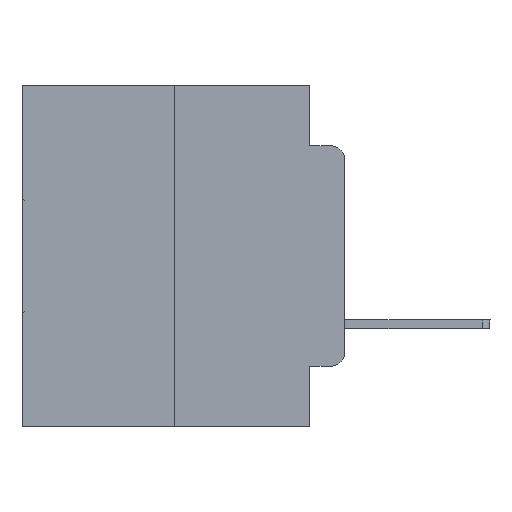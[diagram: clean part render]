
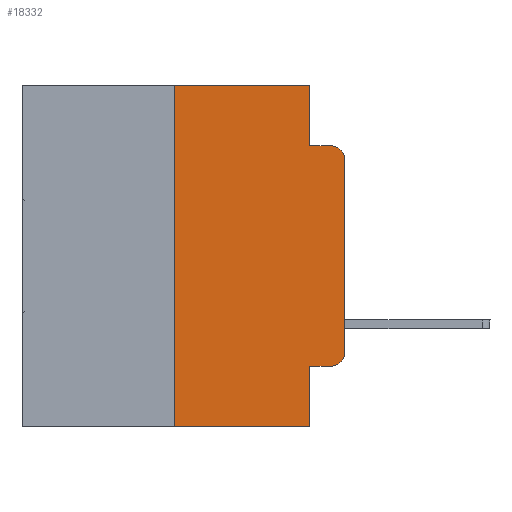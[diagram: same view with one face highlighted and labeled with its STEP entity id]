
A CAD part, left-side view. The second image highlights one B-rep face of the part: STEP entity #18332.
In plain terms, the highlighted planar face has unit normal (-1, 0, 0).
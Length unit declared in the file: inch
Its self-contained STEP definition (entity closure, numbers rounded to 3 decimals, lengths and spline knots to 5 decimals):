
#1055 = ORIENTED_EDGE ( 'NONE', *, *, #14355, .T. ) ;
#1370 = ORIENTED_EDGE ( 'NONE', *, *, #20390, .F. ) ;
#1489 = LINE ( 'NONE', #26837, #17489 ) ;
#1559 = VERTEX_POINT ( 'NONE', #23065 ) ;
#1887 = CARTESIAN_POINT ( 'NONE',  ( 0., 0.051, -0.4115 ) ) ;
#1911 = EDGE_CURVE ( 'NONE', #10479, #4880, #21654, .T. ) ;
#2182 = DIRECTION ( 'NONE',  ( 0., 0., -1. ) ) ;
#3008 = FACE_OUTER_BOUND ( 'NONE', #17630, .T. ) ;
#3124 = DIRECTION ( 'NONE',  ( 0., 0., -1. ) ) ;
#3293 = DIRECTION ( 'NONE',  ( 0., -1., 0. ) ) ;
#3843 = ORIENTED_EDGE ( 'NONE', *, *, #15880, .T. ) ;
#4880 = VERTEX_POINT ( 'NONE', #10643 ) ;
#5521 = CARTESIAN_POINT ( 'NONE',  ( 0., 0.051, -0.5 ) ) ;
#5794 = DIRECTION ( 'NONE',  ( 0., 0., 1. ) ) ;
#5913 = CARTESIAN_POINT ( 'NONE',  ( 0., 0., -0.1085 ) ) ;
#6404 = CARTESIAN_POINT ( 'NONE',  ( 0., 0.02, -0.1085 ) ) ;
#6795 = LINE ( 'NONE', #13493, #24211 ) ;
#7030 = DIRECTION ( 'NONE',  ( 1., 0., 0. ) ) ;
#7141 = DIRECTION ( 'NONE',  ( 0., -1., 0. ) ) ;
#7859 = ORIENTED_EDGE ( 'NONE', *, *, #23474, .F. ) ;
#8102 = AXIS2_PLACEMENT_3D ( 'NONE', #24826, #7030, #2182 ) ;
#8196 = ORIENTED_EDGE ( 'NONE', *, *, #9827, .F. ) ;
#8483 = EDGE_CURVE ( 'NONE', #16882, #14150, #1489, .T. ) ;
#8711 = DIRECTION ( 'NONE',  ( -1., 0., 0. ) ) ;
#9406 = VERTEX_POINT ( 'NONE', #26937 ) ;
#9827 = EDGE_CURVE ( 'NONE', #4880, #22432, #14469, .T. ) ;
#10022 = VECTOR ( 'NONE', #5794, 39.37008 ) ;
#10479 = VERTEX_POINT ( 'NONE', #19181 ) ;
#10643 = CARTESIAN_POINT ( 'NONE',  ( 0., 0.051, -0.0885 ) ) ;
#11920 = VERTEX_POINT ( 'NONE', #29093 ) ;
#12376 = CARTESIAN_POINT ( 'NONE',  ( 0., 0., 0. ) ) ;
#12474 = DIRECTION ( 'NONE',  ( 0., -1., 0. ) ) ;
#12722 = VECTOR ( 'NONE', #7141, 39.37008 ) ;
#12760 = ORIENTED_EDGE ( 'NONE', *, *, #19668, .T. ) ;
#12940 = DIRECTION ( 'NONE',  ( 0., 0., -1. ) ) ;
#13493 = CARTESIAN_POINT ( 'NONE',  ( 0., 0.051, 0. ) ) ;
#14150 = VERTEX_POINT ( 'NONE', #21867 ) ;
#14355 = EDGE_CURVE ( 'NONE', #11920, #16668, #24159, .T. ) ;
#14469 = LINE ( 'NONE', #20763, #12722 ) ;
#14696 = ORIENTED_EDGE ( 'NONE', *, *, #1911, .F. ) ;
#15263 = DIRECTION ( 'NONE',  ( 0., -1., 0. ) ) ;
#15433 = VERTEX_POINT ( 'NONE', #5521 ) ;
#15880 = EDGE_CURVE ( 'NONE', #16668, #22432, #24783, .T. ) ;
#16668 = VERTEX_POINT ( 'NONE', #5913 ) ;
#16882 = VERTEX_POINT ( 'NONE', #1887 ) ;
#17130 = CARTESIAN_POINT ( 'NONE',  ( 0., 0.25, 0. ) ) ;
#17324 = ORIENTED_EDGE ( 'NONE', *, *, #8483, .T. ) ;
#17489 = VECTOR ( 'NONE', #15263, 39.37008 ) ;
#17528 = ORIENTED_EDGE ( 'NONE', *, *, #24005, .F. ) ;
#17630 = EDGE_LOOP ( 'NONE', ( #1055, #3843, #8196, #14696, #17528, #7859, #12760, #1370, #17324, #22551 ) ) ;
#18091 = PLANE ( 'NONE',  #8102 ) ;
#18212 = AXIS2_PLACEMENT_3D ( 'NONE', #25520, #18786, #21042 ) ;
#18332 = ADVANCED_FACE ( 'NONE', ( #3008 ), #18091, .F. ) ;
#18786 = DIRECTION ( 'NONE',  ( -1., 0., 0. ) ) ;
#18971 = CIRCLE ( 'NONE', #18212, 0.02 ) ;
#19181 = CARTESIAN_POINT ( 'NONE',  ( 0., 0.051, 0. ) ) ;
#19240 = LINE ( 'NONE', #17130, #10022 ) ;
#19377 = CARTESIAN_POINT ( 'NONE',  ( 0., 0.473, 0. ) ) ;
#19668 = EDGE_CURVE ( 'NONE', #1559, #15433, #24613, .T. ) ;
#20390 = EDGE_CURVE ( 'NONE', #16882, #15433, #6795, .T. ) ;
#20763 = CARTESIAN_POINT ( 'NONE',  ( 0., 0.051, -0.0885 ) ) ;
#20944 = VECTOR ( 'NONE', #28196, 39.37008 ) ;
#20953 = VECTOR ( 'NONE', #12940, 39.37008 ) ;
#21042 = DIRECTION ( 'NONE',  ( 0., 0., -1. ) ) ;
#21654 = LINE ( 'NONE', #24054, #20953 ) ;
#21665 = LINE ( 'NONE', #19377, #24176 ) ;
#21867 = CARTESIAN_POINT ( 'NONE',  ( 0., 0.02, -0.4115 ) ) ;
#22400 = DIRECTION ( 'NONE',  ( 0., 0., -1. ) ) ;
#22432 = VERTEX_POINT ( 'NONE', #28434 ) ;
#22551 = ORIENTED_EDGE ( 'NONE', *, *, #29241, .T. ) ;
#23065 = CARTESIAN_POINT ( 'NONE',  ( 0., 0.25, -0.5 ) ) ;
#23474 = EDGE_CURVE ( 'NONE', #1559, #9406, #19240, .T. ) ;
#24005 = EDGE_CURVE ( 'NONE', #9406, #10479, #21665, .T. ) ;
#24054 = CARTESIAN_POINT ( 'NONE',  ( 0., 0.051, 0. ) ) ;
#24159 = LINE ( 'NONE', #12376, #20944 ) ;
#24176 = VECTOR ( 'NONE', #3293, 39.37008 ) ;
#24211 = VECTOR ( 'NONE', #3124, 39.37008 ) ;
#24613 = LINE ( 'NONE', #28291, #24941 ) ;
#24783 = CIRCLE ( 'NONE', #24968, 0.02 ) ;
#24826 = CARTESIAN_POINT ( 'NONE',  ( 0., 0.473, 0. ) ) ;
#24941 = VECTOR ( 'NONE', #12474, 39.37008 ) ;
#24968 = AXIS2_PLACEMENT_3D ( 'NONE', #6404, #8711, #22400 ) ;
#25520 = CARTESIAN_POINT ( 'NONE',  ( 0., 0.02, -0.3915 ) ) ;
#26837 = CARTESIAN_POINT ( 'NONE',  ( 0., 0.051, -0.4115 ) ) ;
#26937 = CARTESIAN_POINT ( 'NONE',  ( 0., 0.25, 0. ) ) ;
#28196 = DIRECTION ( 'NONE',  ( 0., 0., 1. ) ) ;
#28291 = CARTESIAN_POINT ( 'NONE',  ( 0., 0.473, -0.5 ) ) ;
#28434 = CARTESIAN_POINT ( 'NONE',  ( 0., 0.02, -0.0885 ) ) ;
#29093 = CARTESIAN_POINT ( 'NONE',  ( 0., 0., -0.3915 ) ) ;
#29241 = EDGE_CURVE ( 'NONE', #14150, #11920, #18971, .T. ) ;
